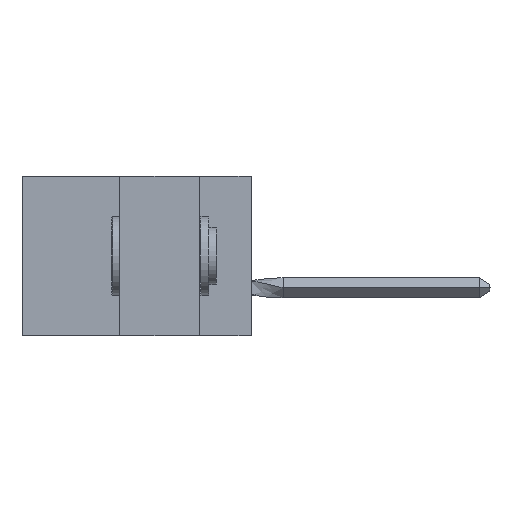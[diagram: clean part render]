
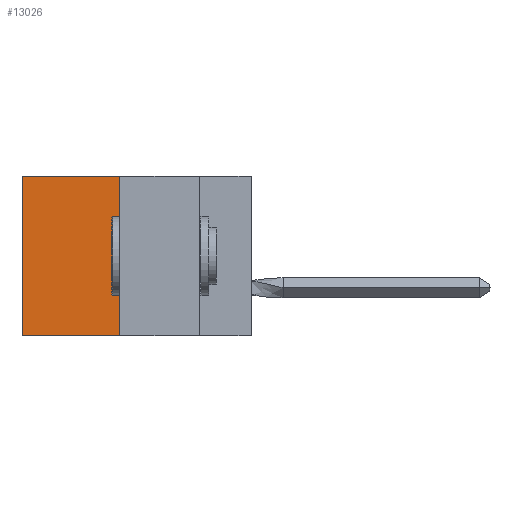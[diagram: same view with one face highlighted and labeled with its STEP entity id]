
A CAD part, left-side view. The second image highlights one B-rep face of the part: STEP entity #13026.
In plain terms, the highlighted planar face has unit normal (-1, 0, 0).
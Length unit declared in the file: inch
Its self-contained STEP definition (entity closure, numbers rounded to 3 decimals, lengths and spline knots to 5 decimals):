
#748 = VERTEX_POINT ( 'NONE', #23703 ) ;
#1362 = EDGE_CURVE ( 'NONE', #21856, #8637, #10669, .T. ) ;
#1399 = VERTEX_POINT ( 'NONE', #6037 ) ;
#2190 = ORIENTED_EDGE ( 'NONE', *, *, #9758, .F. ) ;
#2419 = FACE_OUTER_BOUND ( 'NONE', #8021, .T. ) ;
#3876 = DIRECTION ( 'NONE',  ( 0., 0., -1. ) ) ;
#4348 = DIRECTION ( 'NONE',  ( 1., 0., 0. ) ) ;
#5391 = VECTOR ( 'NONE', #3876, 39.37008 ) ;
#5420 = LINE ( 'NONE', #16635, #25373 ) ;
#6037 = CARTESIAN_POINT ( 'NONE',  ( 0.305, 0.413, -0.5 ) ) ;
#7039 = VECTOR ( 'NONE', #8045, 39.37008 ) ;
#7972 = CARTESIAN_POINT ( 'NONE',  ( 0.305, 0.72, -0.5 ) ) ;
#8021 = EDGE_LOOP ( 'NONE', ( #13884, #18287, #2190, #9444 ) ) ;
#8045 = DIRECTION ( 'NONE',  ( 0., 1., 0. ) ) ;
#8204 = EDGE_CURVE ( 'NONE', #1399, #8637, #14527, .T. ) ;
#8637 = VERTEX_POINT ( 'NONE', #25832 ) ;
#9444 = ORIENTED_EDGE ( 'NONE', *, *, #10090, .T. ) ;
#9565 = CARTESIAN_POINT ( 'NONE',  ( 0.305, 0.413, 0. ) ) ;
#9758 = EDGE_CURVE ( 'NONE', #748, #1399, #5420, .T. ) ;
#10090 = EDGE_CURVE ( 'NONE', #748, #21856, #22217, .T. ) ;
#10669 = LINE ( 'NONE', #7972, #5391 ) ;
#13026 = ADVANCED_FACE ( 'NONE', ( #2419 ), #24214, .F. ) ;
#13884 = ORIENTED_EDGE ( 'NONE', *, *, #1362, .T. ) ;
#14527 = LINE ( 'NONE', #18035, #7039 ) ;
#16254 = CARTESIAN_POINT ( 'NONE',  ( 0.305, 0.413, -0.5 ) ) ;
#16340 = DIRECTION ( 'NONE',  ( 0., 0., -1. ) ) ;
#16456 = AXIS2_PLACEMENT_3D ( 'NONE', #16254, #4348, #16340 ) ;
#16635 = CARTESIAN_POINT ( 'NONE',  ( 0.305, 0.413, -0.5 ) ) ;
#18035 = CARTESIAN_POINT ( 'NONE',  ( 0.305, 0.413, -0.5 ) ) ;
#18287 = ORIENTED_EDGE ( 'NONE', *, *, #8204, .F. ) ;
#19861 = CARTESIAN_POINT ( 'NONE',  ( 0.305, 0.72, 0. ) ) ;
#21762 = DIRECTION ( 'NONE',  ( 0., 1., 0. ) ) ;
#21856 = VERTEX_POINT ( 'NONE', #19861 ) ;
#22217 = LINE ( 'NONE', #9565, #25019 ) ;
#23101 = DIRECTION ( 'NONE',  ( 0., 0., -1. ) ) ;
#23703 = CARTESIAN_POINT ( 'NONE',  ( 0.305, 0.413, 0. ) ) ;
#24214 = PLANE ( 'NONE',  #16456 ) ;
#25019 = VECTOR ( 'NONE', #21762, 39.37008 ) ;
#25373 = VECTOR ( 'NONE', #23101, 39.37008 ) ;
#25832 = CARTESIAN_POINT ( 'NONE',  ( 0.305, 0.72, -0.5 ) ) ;
